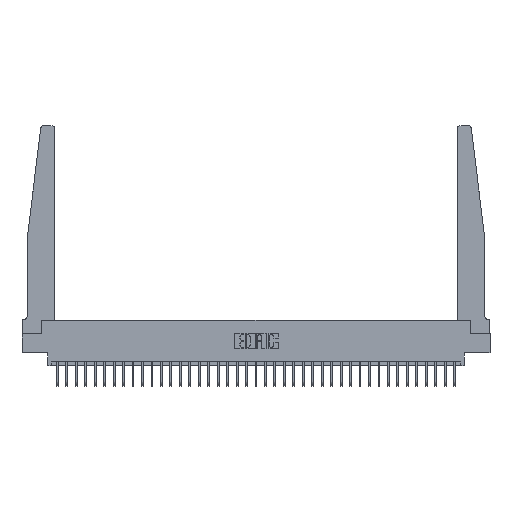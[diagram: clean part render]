
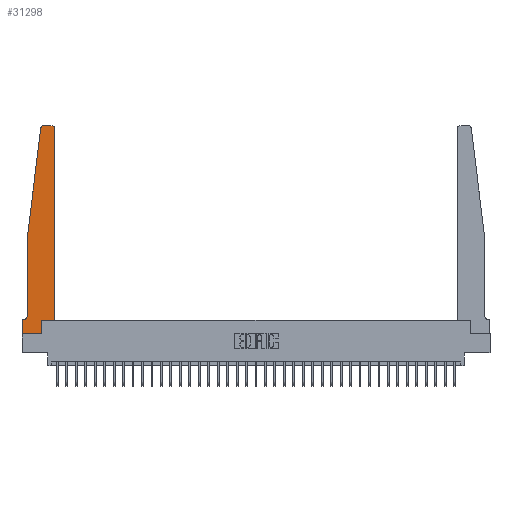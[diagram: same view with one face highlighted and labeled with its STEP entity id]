
A CAD part, top view. The second image highlights one B-rep face of the part: STEP entity #31298.
In plain terms, the highlighted planar face has unit normal (0, 0, 1).
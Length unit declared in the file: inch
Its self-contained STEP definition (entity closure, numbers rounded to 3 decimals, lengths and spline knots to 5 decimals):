
#237 = DIRECTION ( 'NONE',  ( 0., -1., 0. ) ) ;
#386 = EDGE_CURVE ( 'NONE', #25952, #13334, #15049, .T. ) ;
#585 = CARTESIAN_POINT ( 'NONE',  ( 0., 0., 0.37 ) ) ;
#701 = EDGE_CURVE ( 'NONE', #24536, #7946, #9638, .T. ) ;
#1448 = CARTESIAN_POINT ( 'NONE',  ( 0.2605, 0.18, 0.37 ) ) ;
#2117 = VECTOR ( 'NONE', #31452, 39.37008 ) ;
#2876 = CARTESIAN_POINT ( 'NONE',  ( 0., 0.1875, 0.37 ) ) ;
#3888 = DIRECTION ( 'NONE',  ( -1., 0., 0. ) ) ;
#4218 = LINE ( 'NONE', #34017, #2117 ) ;
#4823 = CARTESIAN_POINT ( 'NONE',  ( 0.395, 2.72, 0.37 ) ) ;
#4875 = ORIENTED_EDGE ( 'NONE', *, *, #25680, .T. ) ;
#5000 = CARTESIAN_POINT ( 'NONE',  ( 0.27653, 2.72, 0.37 ) ) ;
#5805 = PLANE ( 'NONE',  #21664 ) ;
#6457 = CARTESIAN_POINT ( 'NONE',  ( 0.015, 0.2375, 0.37 ) ) ;
#7236 = CIRCLE ( 'NONE', #13199, 0.05 ) ;
#7584 = DIRECTION ( 'NONE',  ( 0., 0., 1. ) ) ;
#7946 = VERTEX_POINT ( 'NONE', #17982 ) ;
#8272 = CARTESIAN_POINT ( 'NONE',  ( 0.425, 0.18, 0.37 ) ) ;
#8426 = EDGE_LOOP ( 'NONE', ( #30271, #25336, #23629, #24375, #11750, #24841, #4875, #26524, #30551, #20064, #18211, #27309 ) ) ;
#9414 = DIRECTION ( 'NONE',  ( 0., 0., -1. ) ) ;
#9638 = LINE ( 'NONE', #11019, #25991 ) ;
#9874 = DIRECTION ( 'NONE',  ( 0., 0., 1. ) ) ;
#11019 = CARTESIAN_POINT ( 'NONE',  ( 0.065, 0.1875, 0.37 ) ) ;
#11750 = ORIENTED_EDGE ( 'NONE', *, *, #24063, .T. ) ;
#12168 = LINE ( 'NONE', #585, #25591 ) ;
#12856 = CARTESIAN_POINT ( 'NONE',  ( 0.065, 1.25, 0.37 ) ) ;
#13199 = AXIS2_PLACEMENT_3D ( 'NONE', #6457, #9414, #3888 ) ;
#13334 = VERTEX_POINT ( 'NONE', #12856 ) ;
#13732 = EDGE_CURVE ( 'NONE', #16693, #25952, #15898, .T. ) ;
#13770 = CARTESIAN_POINT ( 'NONE',  ( 0.425, 0.18, 0.37 ) ) ;
#13897 = VECTOR ( 'NONE', #28703, 39.37008 ) ;
#14065 = CARTESIAN_POINT ( 'NONE',  ( 0.065, 0.2375, 0.37 ) ) ;
#14382 = AXIS2_PLACEMENT_3D ( 'NONE', #5000, #7584, #23393 ) ;
#14786 = VERTEX_POINT ( 'NONE', #33966 ) ;
#14808 = FACE_OUTER_BOUND ( 'NONE', #8426, .T. ) ;
#14811 = EDGE_CURVE ( 'NONE', #13334, #16593, #17285, .T. ) ;
#14894 = VECTOR ( 'NONE', #23937, 39.37008 ) ;
#15020 = DIRECTION ( 'NONE',  ( -1., 0., 0. ) ) ;
#15049 = LINE ( 'NONE', #25025, #24716 ) ;
#15304 = CARTESIAN_POINT ( 'NONE',  ( 0.065, 1.25, 0.37 ) ) ;
#15898 = CIRCLE ( 'NONE', #14382, 0.03 ) ;
#16030 = CARTESIAN_POINT ( 'NONE',  ( 0., 0., 0.37 ) ) ;
#16194 = CARTESIAN_POINT ( 'NONE',  ( 0.27653, 2.75, 0.37 ) ) ;
#16309 = DIRECTION ( 'NONE',  ( 1., 0., 0. ) ) ;
#16348 = VERTEX_POINT ( 'NONE', #1448 ) ;
#16593 = VERTEX_POINT ( 'NONE', #14065 ) ;
#16693 = VERTEX_POINT ( 'NONE', #16194 ) ;
#17285 = LINE ( 'NONE', #15304, #13897 ) ;
#17736 = EDGE_CURVE ( 'NONE', #16348, #21860, #4218, .T. ) ;
#17883 = VECTOR ( 'NONE', #21656, 39.37008 ) ;
#17982 = CARTESIAN_POINT ( 'NONE',  ( 0., 0.1875, 0.37 ) ) ;
#18211 = ORIENTED_EDGE ( 'NONE', *, *, #20403, .T. ) ;
#20064 = ORIENTED_EDGE ( 'NONE', *, *, #17736, .T. ) ;
#20403 = EDGE_CURVE ( 'NONE', #21860, #33559, #21218, .T. ) ;
#21218 = LINE ( 'NONE', #8272, #33817 ) ;
#21589 = LINE ( 'NONE', #24271, #14894 ) ;
#21656 = DIRECTION ( 'NONE',  ( 0., 1., 0. ) ) ;
#21664 = AXIS2_PLACEMENT_3D ( 'NONE', #2876, #29723, #16309 ) ;
#21860 = VERTEX_POINT ( 'NONE', #13770 ) ;
#22457 = EDGE_CURVE ( 'NONE', #23517, #16693, #32091, .T. ) ;
#23393 = DIRECTION ( 'NONE',  ( 1., 0., 0. ) ) ;
#23517 = VERTEX_POINT ( 'NONE', #30990 ) ;
#23578 = CARTESIAN_POINT ( 'NONE',  ( 0.425, 2.72, 0.37 ) ) ;
#23629 = ORIENTED_EDGE ( 'NONE', *, *, #386, .T. ) ;
#23937 = DIRECTION ( 'NONE',  ( 1., 0., 0. ) ) ;
#24063 = EDGE_CURVE ( 'NONE', #16593, #24536, #7236, .T. ) ;
#24271 = CARTESIAN_POINT ( 'NONE',  ( 0., 0., 0.37 ) ) ;
#24375 = ORIENTED_EDGE ( 'NONE', *, *, #14811, .T. ) ;
#24536 = VERTEX_POINT ( 'NONE', #25509 ) ;
#24716 = VECTOR ( 'NONE', #33011, 39.37008 ) ;
#24841 = ORIENTED_EDGE ( 'NONE', *, *, #701, .T. ) ;
#25025 = CARTESIAN_POINT ( 'NONE',  ( 0.065, 1.25, 0.37 ) ) ;
#25336 = ORIENTED_EDGE ( 'NONE', *, *, #13732, .T. ) ;
#25435 = DIRECTION ( 'NONE',  ( -1., 0., 0. ) ) ;
#25509 = CARTESIAN_POINT ( 'NONE',  ( 0.015, 0.1875, 0.37 ) ) ;
#25534 = VERTEX_POINT ( 'NONE', #16030 ) ;
#25591 = VECTOR ( 'NONE', #237, 39.37008 ) ;
#25680 = EDGE_CURVE ( 'NONE', #7946, #25534, #12168, .T. ) ;
#25925 = EDGE_CURVE ( 'NONE', #33559, #23517, #30585, .T. ) ;
#25952 = VERTEX_POINT ( 'NONE', #26040 ) ;
#25991 = VECTOR ( 'NONE', #25435, 39.37008 ) ;
#26040 = CARTESIAN_POINT ( 'NONE',  ( 0.24675, 2.72367, 0.37 ) ) ;
#26222 = VECTOR ( 'NONE', #15020, 39.37008 ) ;
#26524 = ORIENTED_EDGE ( 'NONE', *, *, #29946, .T. ) ;
#26968 = CARTESIAN_POINT ( 'NONE',  ( 0.2605, 0.18, 0.37 ) ) ;
#27027 = DIRECTION ( 'NONE',  ( 0., 1., 0. ) ) ;
#27245 = EDGE_CURVE ( 'NONE', #14786, #16348, #29207, .T. ) ;
#27309 = ORIENTED_EDGE ( 'NONE', *, *, #25925, .T. ) ;
#28703 = DIRECTION ( 'NONE',  ( 0., -1., 0. ) ) ;
#28959 = DIRECTION ( 'NONE',  ( 1., 0., 0. ) ) ;
#29207 = LINE ( 'NONE', #26968, #17883 ) ;
#29723 = DIRECTION ( 'NONE',  ( 0., 0., 1. ) ) ;
#29946 = EDGE_CURVE ( 'NONE', #25534, #14786, #21589, .T. ) ;
#30271 = ORIENTED_EDGE ( 'NONE', *, *, #22457, .T. ) ;
#30551 = ORIENTED_EDGE ( 'NONE', *, *, #27245, .T. ) ;
#30585 = CIRCLE ( 'NONE', #34337, 0.03 ) ;
#30990 = CARTESIAN_POINT ( 'NONE',  ( 0.395, 2.75, 0.37 ) ) ;
#31298 = ADVANCED_FACE ( 'NONE', ( #14808 ), #5805, .T. ) ;
#31452 = DIRECTION ( 'NONE',  ( 1., 0., 0. ) ) ;
#32091 = LINE ( 'NONE', #33787, #26222 ) ;
#33011 = DIRECTION ( 'NONE',  ( -0.122, -0.992, 0. ) ) ;
#33559 = VERTEX_POINT ( 'NONE', #23578 ) ;
#33787 = CARTESIAN_POINT ( 'NONE',  ( 0.25, 2.75, 0.37 ) ) ;
#33817 = VECTOR ( 'NONE', #27027, 39.37008 ) ;
#33966 = CARTESIAN_POINT ( 'NONE',  ( 0.2605, 0., 0.37 ) ) ;
#34017 = CARTESIAN_POINT ( 'NONE',  ( 0.425, 0.18, 0.37 ) ) ;
#34337 = AXIS2_PLACEMENT_3D ( 'NONE', #4823, #9874, #28959 ) ;
